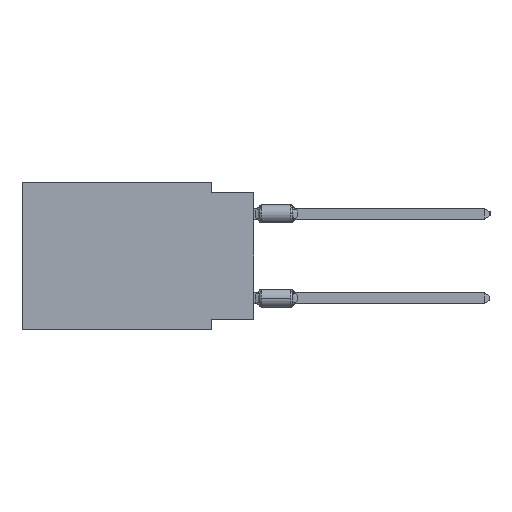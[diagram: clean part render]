
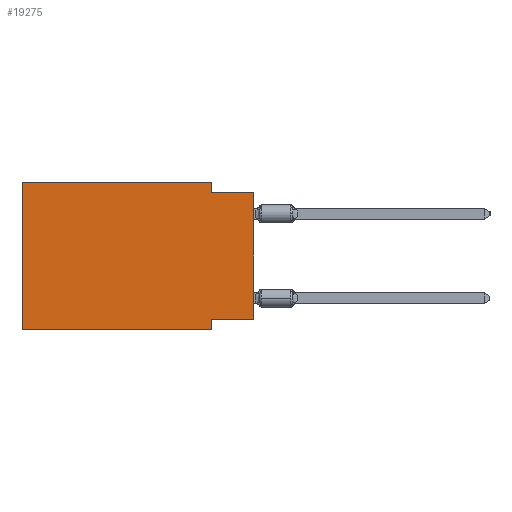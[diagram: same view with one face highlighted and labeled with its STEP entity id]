
A CAD part, left-side view. The second image highlights one B-rep face of the part: STEP entity #19275.
In plain terms, the highlighted planar face has unit normal (-1, 0, 0).
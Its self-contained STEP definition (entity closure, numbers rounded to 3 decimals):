
#277 = VERTEX_POINT ( 'NONE', #28969 ) ;
#666 = VERTEX_POINT ( 'NONE', #12238 ) ;
#1940 = CARTESIAN_POINT ( 'NONE',  ( 0., 2.54, -8.89 ) ) ;
#2176 = VECTOR ( 'NONE', #36693, 1000. ) ;
#3662 = EDGE_CURVE ( 'NONE', #5784, #20898, #25414, .T. ) ;
#4791 = LINE ( 'NONE', #16151, #2176 ) ;
#5425 = CARTESIAN_POINT ( 'NONE',  ( 0., 13.97, 0. ) ) ;
#5784 = VERTEX_POINT ( 'NONE', #21835 ) ;
#6577 = DIRECTION ( 'NONE',  ( 0., 0., -1. ) ) ;
#6668 = EDGE_CURVE ( 'NONE', #20898, #277, #42707, .T. ) ;
#9928 = LINE ( 'NONE', #13635, #32957 ) ;
#11519 = VERTEX_POINT ( 'NONE', #22648 ) ;
#12238 = CARTESIAN_POINT ( 'NONE',  ( 0., 2.54, -8.255 ) ) ;
#12505 = EDGE_CURVE ( 'NONE', #26657, #39993, #23242, .T. ) ;
#12742 = ORIENTED_EDGE ( 'NONE', *, *, #19903, .F. ) ;
#12870 = ORIENTED_EDGE ( 'NONE', *, *, #39419, .F. ) ;
#13635 = CARTESIAN_POINT ( 'NONE',  ( 0., 13.97, -8.89 ) ) ;
#15087 = CARTESIAN_POINT ( 'NONE',  ( 0., 0., 0. ) ) ;
#15560 = ORIENTED_EDGE ( 'NONE', *, *, #44570, .F. ) ;
#16151 = CARTESIAN_POINT ( 'NONE',  ( 0., 0., -8.255 ) ) ;
#17248 = DIRECTION ( 'NONE',  ( 0., -1., 0. ) ) ;
#17567 = DIRECTION ( 'NONE',  ( 1., 0., 0. ) ) ;
#17976 = CARTESIAN_POINT ( 'NONE',  ( 0., 0., -8.255 ) ) ;
#19275 = ADVANCED_FACE ( 'NONE', ( #38365 ), #46020, .F. ) ;
#19903 = EDGE_CURVE ( 'NONE', #26657, #666, #4791, .T. ) ;
#20002 = ORIENTED_EDGE ( 'NONE', *, *, #6668, .F. ) ;
#20898 = VERTEX_POINT ( 'NONE', #51468 ) ;
#21835 = CARTESIAN_POINT ( 'NONE',  ( 0., 13.97, 0. ) ) ;
#22097 = CARTESIAN_POINT ( 'NONE',  ( 0., 13.97, 0. ) ) ;
#22573 = DIRECTION ( 'NONE',  ( 0., 0., -1. ) ) ;
#22630 = DIRECTION ( 'NONE',  ( 0., 0., 1. ) ) ;
#22648 = CARTESIAN_POINT ( 'NONE',  ( 0., 13.97, -8.89 ) ) ;
#23242 = LINE ( 'NONE', #15087, #40574 ) ;
#23480 = LINE ( 'NONE', #35328, #35812 ) ;
#25414 = LINE ( 'NONE', #33323, #44984 ) ;
#26312 = LINE ( 'NONE', #22097, #29643 ) ;
#26428 = ORIENTED_EDGE ( 'NONE', *, *, #3662, .F. ) ;
#26657 = VERTEX_POINT ( 'NONE', #17976 ) ;
#27418 = AXIS2_PLACEMENT_3D ( 'NONE', #5425, #17567, #22573 ) ;
#27461 = EDGE_CURVE ( 'NONE', #11519, #46679, #9928, .T. ) ;
#27941 = ORIENTED_EDGE ( 'NONE', *, *, #12505, .T. ) ;
#28969 = CARTESIAN_POINT ( 'NONE',  ( 0., 2.54, -0.635 ) ) ;
#29643 = VECTOR ( 'NONE', #22630, 1000. ) ;
#30235 = DIRECTION ( 'NONE',  ( 0., -1., 0. ) ) ;
#30417 = LINE ( 'NONE', #1940, #39270 ) ;
#31555 = ORIENTED_EDGE ( 'NONE', *, *, #32030, .F. ) ;
#32030 = EDGE_CURVE ( 'NONE', #11519, #5784, #26312, .T. ) ;
#32183 = DIRECTION ( 'NONE',  ( 0., 0., 1. ) ) ;
#32957 = VECTOR ( 'NONE', #30235, 1000. ) ;
#33323 = CARTESIAN_POINT ( 'NONE',  ( 0., 13.97, 0. ) ) ;
#34141 = EDGE_LOOP ( 'NONE', ( #27941, #12870, #20002, #26428, #31555, #49306, #15560, #12742 ) ) ;
#34527 = CARTESIAN_POINT ( 'NONE',  ( 0., 2.54, 0. ) ) ;
#35070 = DIRECTION ( 'NONE',  ( 0., -1., 0. ) ) ;
#35328 = CARTESIAN_POINT ( 'NONE',  ( 0., 0., -0.635 ) ) ;
#35812 = VECTOR ( 'NONE', #35070, 1000. ) ;
#36693 = DIRECTION ( 'NONE',  ( 0., 1., 0. ) ) ;
#37541 = DIRECTION ( 'NONE',  ( 0., 0., -1. ) ) ;
#38365 = FACE_OUTER_BOUND ( 'NONE', #34141, .T. ) ;
#39270 = VECTOR ( 'NONE', #37541, 1000. ) ;
#39419 = EDGE_CURVE ( 'NONE', #277, #39993, #23480, .T. ) ;
#39993 = VERTEX_POINT ( 'NONE', #44414 ) ;
#40574 = VECTOR ( 'NONE', #32183, 1000. ) ;
#42707 = LINE ( 'NONE', #34527, #51911 ) ;
#44414 = CARTESIAN_POINT ( 'NONE',  ( 0., 0., -0.635 ) ) ;
#44570 = EDGE_CURVE ( 'NONE', #666, #46679, #30417, .T. ) ;
#44984 = VECTOR ( 'NONE', #17248, 1000. ) ;
#46020 = PLANE ( 'NONE',  #27418 ) ;
#46679 = VERTEX_POINT ( 'NONE', #48374 ) ;
#48374 = CARTESIAN_POINT ( 'NONE',  ( 0., 2.54, -8.89 ) ) ;
#49306 = ORIENTED_EDGE ( 'NONE', *, *, #27461, .T. ) ;
#51468 = CARTESIAN_POINT ( 'NONE',  ( 0., 2.54, 0. ) ) ;
#51911 = VECTOR ( 'NONE', #6577, 1000. ) ;
